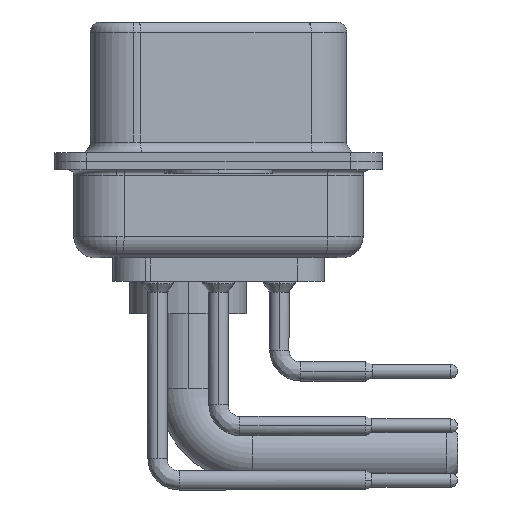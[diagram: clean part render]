
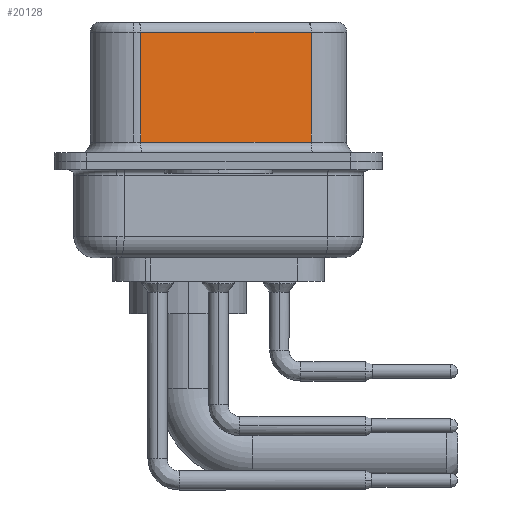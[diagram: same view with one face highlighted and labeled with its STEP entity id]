
A CAD part, left-side view. The second image highlights one B-rep face of the part: STEP entity #20128.
In plain terms, the highlighted planar face has unit normal (-0.985, -0.174, 0).
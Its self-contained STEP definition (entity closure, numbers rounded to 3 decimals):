
#87 = LINE ( 'NONE', #10214, #21096 ) ;
#503 = CARTESIAN_POINT ( 'NONE',  ( 5.132, -4.322, 6.02 ) ) ;
#1400 = LINE ( 'NONE', #30164, #9140 ) ;
#1434 = CARTESIAN_POINT ( 'NONE',  ( 5.132, -4.322, 6.02 ) ) ;
#2653 = PLANE ( 'NONE',  #26882 ) ;
#2816 = FACE_OUTER_BOUND ( 'NONE', #20568, .T. ) ;
#5237 = VERTEX_POINT ( 'NONE', #14770 ) ;
#6792 = ORIENTED_EDGE ( 'NONE', *, *, #33081, .T. ) ;
#7967 = VECTOR ( 'NONE', #26060, 1000. ) ;
#8303 = VECTOR ( 'NONE', #33499, 1000. ) ;
#9140 = VECTOR ( 'NONE', #11713, 1000. ) ;
#10214 = CARTESIAN_POINT ( 'NONE',  ( 5.132, -4.322, 0.9 ) ) ;
#11713 = DIRECTION ( 'NONE',  ( 0., 0., -1. ) ) ;
#12949 = ORIENTED_EDGE ( 'NONE', *, *, #14611, .T. ) ;
#13347 = CARTESIAN_POINT ( 'NONE',  ( 3.73, 3.628, 0.9 ) ) ;
#14611 = EDGE_CURVE ( 'NONE', #33369, #15756, #17632, .T. ) ;
#14770 = CARTESIAN_POINT ( 'NONE',  ( 5.132, -4.322, 0.9 ) ) ;
#15515 = ORIENTED_EDGE ( 'NONE', *, *, #27584, .T. ) ;
#15756 = VERTEX_POINT ( 'NONE', #33193 ) ;
#16240 = DIRECTION ( 'NONE',  ( 0.985, 0.174, 0. ) ) ;
#17632 = LINE ( 'NONE', #1434, #8303 ) ;
#18222 = DIRECTION ( 'NONE',  ( 0.174, -0.985, 0. ) ) ;
#18680 = CARTESIAN_POINT ( 'NONE',  ( 5.132, -4.322, 6.52 ) ) ;
#20128 = ADVANCED_FACE ( 'NONE', ( #2816 ), #2653, .F. ) ;
#20568 = EDGE_LOOP ( 'NONE', ( #20832, #12949, #6792, #15515 ) ) ;
#20832 = ORIENTED_EDGE ( 'NONE', *, *, #32459, .F. ) ;
#21096 = VECTOR ( 'NONE', #18222, 1000. ) ;
#26060 = DIRECTION ( 'NONE',  ( 0., 0., -1. ) ) ;
#26222 = CARTESIAN_POINT ( 'NONE',  ( 5.132, -4.322, 6.52 ) ) ;
#26882 = AXIS2_PLACEMENT_3D ( 'NONE', #18680, #16240, #32113 ) ;
#27584 = EDGE_CURVE ( 'NONE', #32415, #5237, #87, .T. ) ;
#30164 = CARTESIAN_POINT ( 'NONE',  ( 3.73, 3.628, 6.52 ) ) ;
#31962 = LINE ( 'NONE', #26222, #7967 ) ;
#32113 = DIRECTION ( 'NONE',  ( -0.174, 0.985, 0. ) ) ;
#32415 = VERTEX_POINT ( 'NONE', #13347 ) ;
#32459 = EDGE_CURVE ( 'NONE', #33369, #5237, #31962, .T. ) ;
#33081 = EDGE_CURVE ( 'NONE', #15756, #32415, #1400, .T. ) ;
#33193 = CARTESIAN_POINT ( 'NONE',  ( 3.73, 3.628, 6.02 ) ) ;
#33369 = VERTEX_POINT ( 'NONE', #503 ) ;
#33499 = DIRECTION ( 'NONE',  ( -0.174, 0.985, 0. ) ) ;
